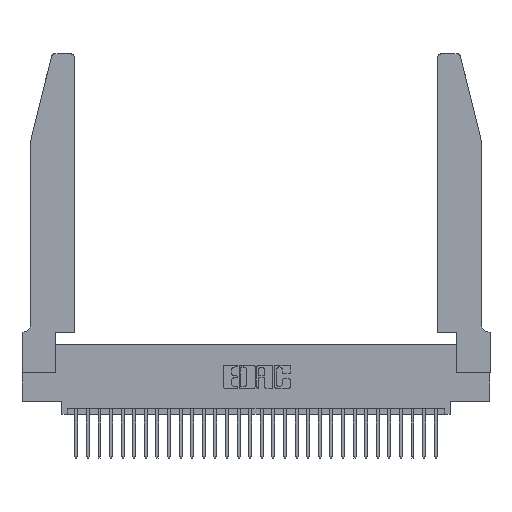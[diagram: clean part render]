
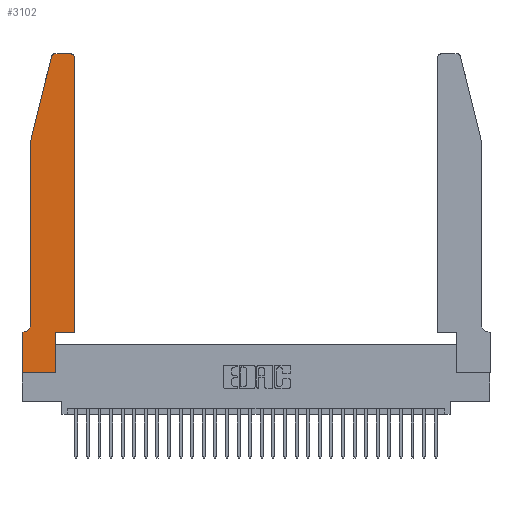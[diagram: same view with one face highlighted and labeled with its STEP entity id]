
A CAD part, top view. The second image highlights one B-rep face of the part: STEP entity #3102.
In plain terms, the highlighted planar face has unit normal (0, 0, 1).
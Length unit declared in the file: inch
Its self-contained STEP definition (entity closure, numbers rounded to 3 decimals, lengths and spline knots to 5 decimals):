
#376 = ORIENTED_EDGE ( 'NONE', *, *, #16578, .T. ) ;
#691 = EDGE_CURVE ( 'NONE', #3557, #29698, #26626, .T. ) ;
#1243 = CARTESIAN_POINT ( 'NONE',  ( 0.2865, 0., 0.37 ) ) ;
#1275 = EDGE_CURVE ( 'NONE', #10858, #10023, #12247, .T. ) ;
#1576 = VECTOR ( 'NONE', #26218, 39.37008 ) ;
#1664 = CARTESIAN_POINT ( 'NONE',  ( 0.4505, 0.35, 0.37 ) ) ;
#1809 = VECTOR ( 'NONE', #9468, 39.37008 ) ;
#1864 = DIRECTION ( 'NONE',  ( -0.239, -0.971, 0. ) ) ;
#2172 = LINE ( 'NONE', #2275, #14366 ) ;
#2211 = DIRECTION ( 'NONE',  ( 0., 0., 1. ) ) ;
#2252 = ORIENTED_EDGE ( 'NONE', *, *, #27249, .T. ) ;
#2275 = CARTESIAN_POINT ( 'NONE',  ( 0.2605, 2.75, 0.37 ) ) ;
#3102 = ADVANCED_FACE ( 'NONE', ( #8331 ), #31205, .T. ) ;
#3255 = CARTESIAN_POINT ( 'NONE',  ( 0.284, 2.75, 0.37 ) ) ;
#3557 = VERTEX_POINT ( 'NONE', #13898 ) ;
#4226 = AXIS2_PLACEMENT_3D ( 'NONE', #19821, #5321, #22242 ) ;
#4637 = CARTESIAN_POINT ( 'NONE',  ( 0.2865, 0.35, 0.37 ) ) ;
#4772 = DIRECTION ( 'NONE',  ( -1., 0., 0. ) ) ;
#5321 = DIRECTION ( 'NONE',  ( 0., 0., -1. ) ) ;
#5730 = CARTESIAN_POINT ( 'NONE',  ( 0., 0., 0.37 ) ) ;
#5797 = VECTOR ( 'NONE', #22637, 39.37008 ) ;
#6201 = DIRECTION ( 'NONE',  ( 0., 0., 1. ) ) ;
#6985 = CARTESIAN_POINT ( 'NONE',  ( 0.4505, 0.35, 0.37 ) ) ;
#7053 = CARTESIAN_POINT ( 'NONE',  ( 0.0755, 0.35, 0.37 ) ) ;
#7203 = EDGE_CURVE ( 'NONE', #13939, #9284, #25579, .T. ) ;
#7311 = LINE ( 'NONE', #5730, #5797 ) ;
#7971 = VERTEX_POINT ( 'NONE', #23479 ) ;
#8331 = FACE_OUTER_BOUND ( 'NONE', #23669, .T. ) ;
#8358 = CIRCLE ( 'NONE', #26146, 0.03 ) ;
#8688 = CARTESIAN_POINT ( 'NONE',  ( 0.4205, 2.72, 0.37 ) ) ;
#9284 = VERTEX_POINT ( 'NONE', #16660 ) ;
#9468 = DIRECTION ( 'NONE',  ( 1., 0., 0. ) ) ;
#9531 = DIRECTION ( 'NONE',  ( -1., 0., 0. ) ) ;
#9699 = CARTESIAN_POINT ( 'NONE',  ( 0.2865, 0.35, 0.37 ) ) ;
#9985 = ORIENTED_EDGE ( 'NONE', *, *, #25851, .T. ) ;
#10023 = VERTEX_POINT ( 'NONE', #1243 ) ;
#10323 = ORIENTED_EDGE ( 'NONE', *, *, #28484, .T. ) ;
#10858 = VERTEX_POINT ( 'NONE', #19066 ) ;
#11543 = EDGE_CURVE ( 'NONE', #11967, #7971, #29000, .T. ) ;
#11544 = DIRECTION ( 'NONE',  ( 1., 0., 0. ) ) ;
#11826 = LINE ( 'NONE', #9699, #24651 ) ;
#11839 = ORIENTED_EDGE ( 'NONE', *, *, #21441, .T. ) ;
#11967 = VERTEX_POINT ( 'NONE', #18248 ) ;
#12074 = AXIS2_PLACEMENT_3D ( 'NONE', #20728, #6201, #23122 ) ;
#12137 = EDGE_CURVE ( 'NONE', #25869, #13939, #18806, .T. ) ;
#12247 = LINE ( 'NONE', #19435, #30709 ) ;
#12422 = EDGE_CURVE ( 'NONE', #9284, #11967, #27086, .T. ) ;
#12526 = VERTEX_POINT ( 'NONE', #3255 ) ;
#13135 = VECTOR ( 'NONE', #1864, 39.37008 ) ;
#13505 = DIRECTION ( 'NONE',  ( 0., -1., 0. ) ) ;
#13898 = CARTESIAN_POINT ( 'NONE',  ( 0.4505, 0.35, 0.37 ) ) ;
#13939 = VERTEX_POINT ( 'NONE', #15045 ) ;
#14011 = CARTESIAN_POINT ( 'NONE',  ( 0.0755, 2., 0.37 ) ) ;
#14038 = EDGE_CURVE ( 'NONE', #7971, #10858, #7311, .T. ) ;
#14312 = DIRECTION ( 'NONE',  ( 0., 1., 0. ) ) ;
#14366 = VECTOR ( 'NONE', #4772, 39.37008 ) ;
#15045 = CARTESIAN_POINT ( 'NONE',  ( 0.0755, 2., 0.37 ) ) ;
#15417 = VECTOR ( 'NONE', #9531, 39.37008 ) ;
#15963 = ORIENTED_EDGE ( 'NONE', *, *, #14038, .T. ) ;
#16578 = EDGE_CURVE ( 'NONE', #21938, #3557, #21198, .T. ) ;
#16660 = CARTESIAN_POINT ( 'NONE',  ( 0.0755, 0.42, 0.37 ) ) ;
#16781 = CARTESIAN_POINT ( 'NONE',  ( 0., 0.35, 0.37 ) ) ;
#17103 = ORIENTED_EDGE ( 'NONE', *, *, #7203, .T. ) ;
#18248 = CARTESIAN_POINT ( 'NONE',  ( 0.0055, 0.35, 0.37 ) ) ;
#18806 = LINE ( 'NONE', #14011, #13135 ) ;
#19003 = ORIENTED_EDGE ( 'NONE', *, *, #12137, .T. ) ;
#19066 = CARTESIAN_POINT ( 'NONE',  ( 0., 0., 0.37 ) ) ;
#19215 = DIRECTION ( 'NONE',  ( 1., 0., 0. ) ) ;
#19435 = CARTESIAN_POINT ( 'NONE',  ( 0., 0., 0.37 ) ) ;
#19821 = CARTESIAN_POINT ( 'NONE',  ( 0.0055, 0.42, 0.37 ) ) ;
#20090 = VERTEX_POINT ( 'NONE', #25769 ) ;
#20709 = VECTOR ( 'NONE', #13505, 39.37008 ) ;
#20728 = CARTESIAN_POINT ( 'NONE',  ( 0.284, 2.72, 0.37 ) ) ;
#21198 = LINE ( 'NONE', #6985, #1809 ) ;
#21441 = EDGE_CURVE ( 'NONE', #10023, #21938, #11826, .T. ) ;
#21938 = VERTEX_POINT ( 'NONE', #4637 ) ;
#22242 = DIRECTION ( 'NONE',  ( -1., 0., 0. ) ) ;
#22637 = DIRECTION ( 'NONE',  ( 0., -1., 0. ) ) ;
#23122 = DIRECTION ( 'NONE',  ( 1., 0., 0. ) ) ;
#23479 = CARTESIAN_POINT ( 'NONE',  ( 0., 0.35, 0.37 ) ) ;
#23520 = ORIENTED_EDGE ( 'NONE', *, *, #12422, .T. ) ;
#23669 = EDGE_LOOP ( 'NONE', ( #2252, #10323, #19003, #17103, #23520, #27305, #15963, #28803, #11839, #376, #26951, #9985 ) ) ;
#23696 = CARTESIAN_POINT ( 'NONE',  ( 0.4505, 2.72, 0.37 ) ) ;
#24651 = VECTOR ( 'NONE', #14312, 39.37008 ) ;
#25579 = LINE ( 'NONE', #27940, #20709 ) ;
#25674 = AXIS2_PLACEMENT_3D ( 'NONE', #16781, #2211, #19215 ) ;
#25769 = CARTESIAN_POINT ( 'NONE',  ( 0.4205, 2.75, 0.37 ) ) ;
#25851 = EDGE_CURVE ( 'NONE', #29698, #20090, #8358, .T. ) ;
#25869 = VERTEX_POINT ( 'NONE', #30815 ) ;
#25979 = DIRECTION ( 'NONE',  ( 0., 0., 1. ) ) ;
#25980 = CIRCLE ( 'NONE', #12074, 0.03 ) ;
#26146 = AXIS2_PLACEMENT_3D ( 'NONE', #8688, #25979, #11544 ) ;
#26218 = DIRECTION ( 'NONE',  ( 0., 1., 0. ) ) ;
#26626 = LINE ( 'NONE', #1664, #1576 ) ;
#26951 = ORIENTED_EDGE ( 'NONE', *, *, #691, .T. ) ;
#27086 = CIRCLE ( 'NONE', #4226, 0.07 ) ;
#27249 = EDGE_CURVE ( 'NONE', #20090, #12526, #2172, .T. ) ;
#27305 = ORIENTED_EDGE ( 'NONE', *, *, #11543, .T. ) ;
#27940 = CARTESIAN_POINT ( 'NONE',  ( 0.0755, 2., 0.37 ) ) ;
#28484 = EDGE_CURVE ( 'NONE', #12526, #25869, #25980, .T. ) ;
#28803 = ORIENTED_EDGE ( 'NONE', *, *, #1275, .T. ) ;
#29000 = LINE ( 'NONE', #7053, #15417 ) ;
#29001 = DIRECTION ( 'NONE',  ( 1., 0., 0. ) ) ;
#29698 = VERTEX_POINT ( 'NONE', #23696 ) ;
#30709 = VECTOR ( 'NONE', #29001, 39.37008 ) ;
#30815 = CARTESIAN_POINT ( 'NONE',  ( 0.25487, 2.72718, 0.37 ) ) ;
#31205 = PLANE ( 'NONE',  #25674 ) ;
